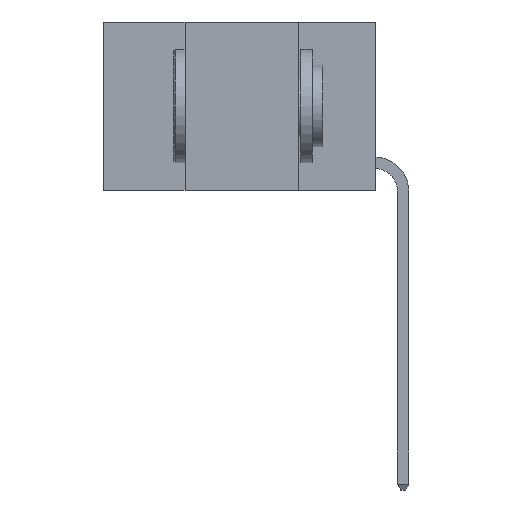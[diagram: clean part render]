
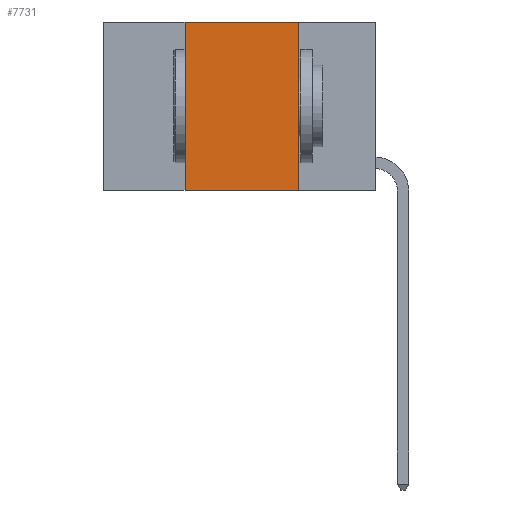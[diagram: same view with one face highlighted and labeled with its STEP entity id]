
A CAD part, left-side view. The second image highlights one B-rep face of the part: STEP entity #7731.
In plain terms, the highlighted planar face has unit normal (-1, 0, 0).
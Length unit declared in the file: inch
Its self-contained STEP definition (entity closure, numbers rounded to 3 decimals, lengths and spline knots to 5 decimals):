
#611 = LINE ( 'NONE', #738, #4578 ) ;
#738 = CARTESIAN_POINT ( 'NONE',  ( 0., 0.6, -0.37 ) ) ;
#1095 = LINE ( 'NONE', #8237, #9071 ) ;
#1224 = LINE ( 'NONE', #9192, #6678 ) ;
#1246 = VERTEX_POINT ( 'NONE', #9018 ) ;
#1250 = PLANE ( 'NONE',  #5110 ) ;
#1357 = CARTESIAN_POINT ( 'NONE',  ( 0., 0.17, 0. ) ) ;
#1990 = LINE ( 'NONE', #2808, #9867 ) ;
#2030 = DIRECTION ( 'NONE',  ( 1., 0., 0. ) ) ;
#2258 = EDGE_LOOP ( 'NONE', ( #8163, #8170, #8179, #8209 ) ) ;
#2808 = CARTESIAN_POINT ( 'NONE',  ( 0., 0.6, 0. ) ) ;
#3100 = CARTESIAN_POINT ( 'NONE',  ( 0., 0.17, -0.37 ) ) ;
#3683 = VERTEX_POINT ( 'NONE', #1357 ) ;
#4464 = DIRECTION ( 'NONE',  ( 0., 0., -1. ) ) ;
#4578 = VECTOR ( 'NONE', #6185, 39.37008 ) ;
#4785 = EDGE_CURVE ( 'NONE', #1246, #3683, #1990, .T. ) ;
#5110 = AXIS2_PLACEMENT_3D ( 'NONE', #9663, #2030, #7442 ) ;
#5123 = FACE_OUTER_BOUND ( 'NONE', #2258, .T. ) ;
#5669 = EDGE_CURVE ( 'NONE', #8798, #8771, #611, .T. ) ;
#6137 = DIRECTION ( 'NONE',  ( 0., 0., 1. ) ) ;
#6161 = EDGE_CURVE ( 'NONE', #8798, #1246, #1224, .T. ) ;
#6185 = DIRECTION ( 'NONE',  ( 0., -1., 0. ) ) ;
#6651 = DIRECTION ( 'NONE',  ( 0., -1., 0. ) ) ;
#6659 = EDGE_CURVE ( 'NONE', #3683, #8771, #1095, .T. ) ;
#6678 = VECTOR ( 'NONE', #6137, 39.37008 ) ;
#7442 = DIRECTION ( 'NONE',  ( 0., 0., -1. ) ) ;
#7731 = ADVANCED_FACE ( 'NONE', ( #5123 ), #1250, .F. ) ;
#8163 = ORIENTED_EDGE ( 'NONE', *, *, #6659, .F. ) ;
#8170 = ORIENTED_EDGE ( 'NONE', *, *, #4785, .F. ) ;
#8179 = ORIENTED_EDGE ( 'NONE', *, *, #6161, .F. ) ;
#8209 = ORIENTED_EDGE ( 'NONE', *, *, #5669, .T. ) ;
#8237 = CARTESIAN_POINT ( 'NONE',  ( 0., 0.17, 0. ) ) ;
#8496 = CARTESIAN_POINT ( 'NONE',  ( 0., 0.42, -0.37 ) ) ;
#8771 = VERTEX_POINT ( 'NONE', #3100 ) ;
#8798 = VERTEX_POINT ( 'NONE', #8496 ) ;
#9018 = CARTESIAN_POINT ( 'NONE',  ( 0., 0.42, 0. ) ) ;
#9071 = VECTOR ( 'NONE', #4464, 39.37008 ) ;
#9192 = CARTESIAN_POINT ( 'NONE',  ( 0., 0.42, 0. ) ) ;
#9663 = CARTESIAN_POINT ( 'NONE',  ( 0., 0.6, 0. ) ) ;
#9867 = VECTOR ( 'NONE', #6651, 39.37008 ) ;
